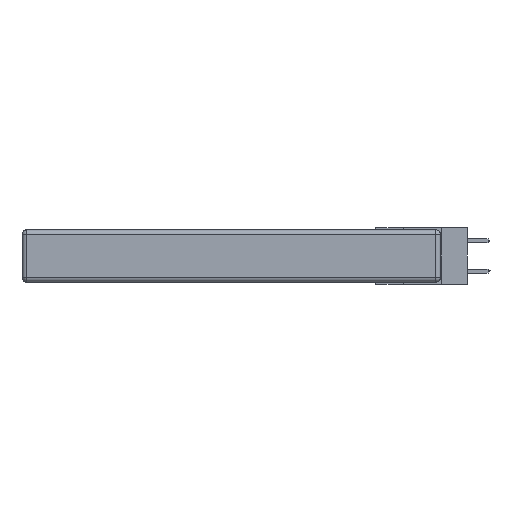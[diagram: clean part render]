
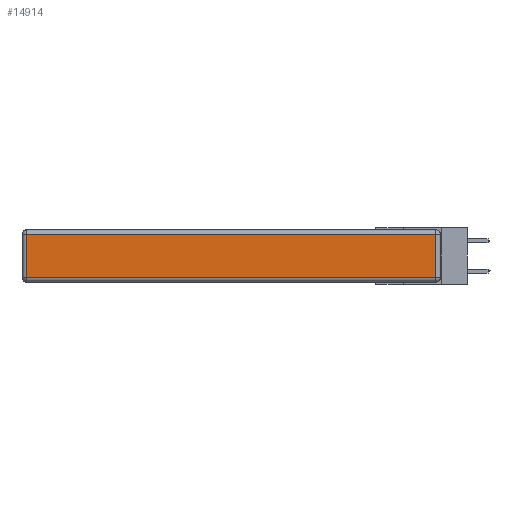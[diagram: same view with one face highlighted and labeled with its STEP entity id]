
A CAD part, left-side view. The second image highlights one B-rep face of the part: STEP entity #14914.
In plain terms, the highlighted planar face has unit normal (-1, 0, 0).
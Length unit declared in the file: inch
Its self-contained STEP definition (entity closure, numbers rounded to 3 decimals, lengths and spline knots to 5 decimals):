
#433 = DIRECTION ( 'NONE',  ( 0., -1., 0. ) ) ;
#835 = ORIENTED_EDGE ( 'NONE', *, *, #3072, .T. ) ;
#1095 = DIRECTION ( 'NONE',  ( 0., 1., 0. ) ) ;
#2027 = AXIS2_PLACEMENT_3D ( 'NONE', #7260, #12068, #14076 ) ;
#2136 = CARTESIAN_POINT ( 'NONE',  ( 0., 0., -0.313 ) ) ;
#2895 = ORIENTED_EDGE ( 'NONE', *, *, #18894, .T. ) ;
#3072 = EDGE_CURVE ( 'NONE', #15945, #19890, #4022, .T. ) ;
#4022 = LINE ( 'NONE', #20520, #6010 ) ;
#4180 = VECTOR ( 'NONE', #1095, 39.37008 ) ;
#5696 = LINE ( 'NONE', #11010, #14665 ) ;
#6010 = VECTOR ( 'NONE', #14529, 39.37008 ) ;
#6223 = CARTESIAN_POINT ( 'NONE',  ( 0., 0.03, -0.03 ) ) ;
#6412 = LINE ( 'NONE', #16717, #4180 ) ;
#7260 = CARTESIAN_POINT ( 'NONE',  ( 0., 0., -0.343 ) ) ;
#8859 = PLANE ( 'NONE',  #2027 ) ;
#9584 = VECTOR ( 'NONE', #433, 39.37008 ) ;
#11010 = CARTESIAN_POINT ( 'NONE',  ( 0., 2.72, -0.343 ) ) ;
#11131 = VERTEX_POINT ( 'NONE', #12479 ) ;
#11354 = DIRECTION ( 'NONE',  ( 0., 0., -1. ) ) ;
#11997 = EDGE_LOOP ( 'NONE', ( #15298, #835, #2895, #12011 ) ) ;
#12011 = ORIENTED_EDGE ( 'NONE', *, *, #20615, .T. ) ;
#12068 = DIRECTION ( 'NONE',  ( -1., 0., 0. ) ) ;
#12479 = CARTESIAN_POINT ( 'NONE',  ( 0., 2.72, -0.03 ) ) ;
#13213 = LINE ( 'NONE', #2136, #9584 ) ;
#14076 = DIRECTION ( 'NONE',  ( 0., 0., 1. ) ) ;
#14529 = DIRECTION ( 'NONE',  ( 0., 0., 1. ) ) ;
#14665 = VECTOR ( 'NONE', #11354, 39.37008 ) ;
#14914 = ADVANCED_FACE ( 'NONE', ( #19507 ), #8859, .T. ) ;
#15298 = ORIENTED_EDGE ( 'NONE', *, *, #16678, .T. ) ;
#15945 = VERTEX_POINT ( 'NONE', #19555 ) ;
#16678 = EDGE_CURVE ( 'NONE', #20159, #15945, #13213, .T. ) ;
#16717 = CARTESIAN_POINT ( 'NONE',  ( 0., 2.75, -0.03 ) ) ;
#18135 = CARTESIAN_POINT ( 'NONE',  ( 0., 2.72, -0.313 ) ) ;
#18894 = EDGE_CURVE ( 'NONE', #19890, #11131, #6412, .T. ) ;
#19507 = FACE_OUTER_BOUND ( 'NONE', #11997, .T. ) ;
#19555 = CARTESIAN_POINT ( 'NONE',  ( 0., 0.03, -0.313 ) ) ;
#19890 = VERTEX_POINT ( 'NONE', #6223 ) ;
#20159 = VERTEX_POINT ( 'NONE', #18135 ) ;
#20520 = CARTESIAN_POINT ( 'NONE',  ( 0., 0.03, -0.343 ) ) ;
#20615 = EDGE_CURVE ( 'NONE', #11131, #20159, #5696, .T. ) ;
